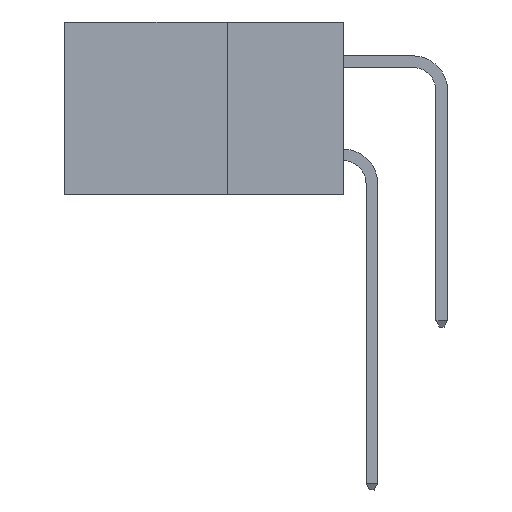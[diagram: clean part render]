
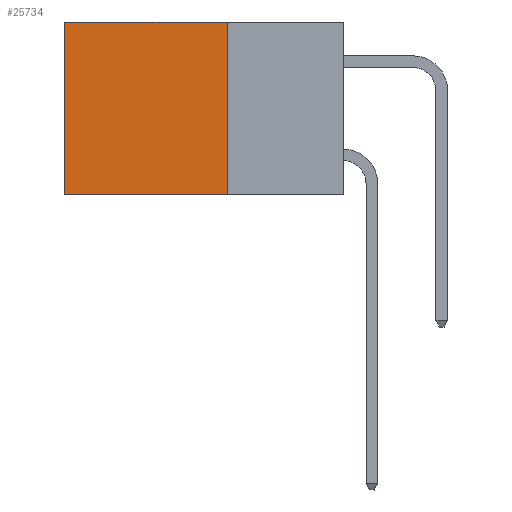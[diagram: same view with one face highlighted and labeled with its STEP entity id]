
A CAD part, left-side view. The second image highlights one B-rep face of the part: STEP entity #25734.
In plain terms, the highlighted planar face has unit normal (-1, 0, 0).
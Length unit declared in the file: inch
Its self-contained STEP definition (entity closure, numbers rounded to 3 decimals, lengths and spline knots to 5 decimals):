
#256 = CARTESIAN_POINT ( 'NONE',  ( 0.298, 0.25, -0.37 ) ) ;
#2157 = CARTESIAN_POINT ( 'NONE',  ( 0.298, 0.6, 0. ) ) ;
#3060 = LINE ( 'NONE', #29448, #22482 ) ;
#4699 = AXIS2_PLACEMENT_3D ( 'NONE', #28687, #28390, #28597 ) ;
#5177 = CARTESIAN_POINT ( 'NONE',  ( 0.298, 0.6, 0. ) ) ;
#5462 = VECTOR ( 'NONE', #14297, 39.37008 ) ;
#5590 = VERTEX_POINT ( 'NONE', #5177 ) ;
#5733 = CARTESIAN_POINT ( 'NONE',  ( 0.298, 0.25, 0. ) ) ;
#6055 = EDGE_CURVE ( 'NONE', #10952, #9444, #3060, .T. ) ;
#7661 = VERTEX_POINT ( 'NONE', #23464 ) ;
#8648 = LINE ( 'NONE', #2157, #25894 ) ;
#9320 = EDGE_LOOP ( 'NONE', ( #13566, #17586, #14301, #10245 ) ) ;
#9444 = VERTEX_POINT ( 'NONE', #256 ) ;
#10245 = ORIENTED_EDGE ( 'NONE', *, *, #13173, .T. ) ;
#10952 = VERTEX_POINT ( 'NONE', #5733 ) ;
#12190 = CARTESIAN_POINT ( 'NONE',  ( 0.298, 0.25, 0. ) ) ;
#12520 = PLANE ( 'NONE',  #4699 ) ;
#13173 = EDGE_CURVE ( 'NONE', #10952, #5590, #18388, .T. ) ;
#13566 = ORIENTED_EDGE ( 'NONE', *, *, #13704, .T. ) ;
#13704 = EDGE_CURVE ( 'NONE', #5590, #7661, #8648, .T. ) ;
#14297 = DIRECTION ( 'NONE',  ( 0., 1., 0. ) ) ;
#14301 = ORIENTED_EDGE ( 'NONE', *, *, #6055, .F. ) ;
#14384 = EDGE_CURVE ( 'NONE', #9444, #7661, #21208, .T. ) ;
#15208 = FACE_OUTER_BOUND ( 'NONE', #9320, .T. ) ;
#16207 = CARTESIAN_POINT ( 'NONE',  ( 0.298, 0.25, -0.37 ) ) ;
#17586 = ORIENTED_EDGE ( 'NONE', *, *, #14384, .F. ) ;
#18014 = DIRECTION ( 'NONE',  ( 0., 0., -1. ) ) ;
#18388 = LINE ( 'NONE', #12190, #5462 ) ;
#21208 = LINE ( 'NONE', #16207, #26947 ) ;
#22482 = VECTOR ( 'NONE', #18014, 39.37008 ) ;
#23464 = CARTESIAN_POINT ( 'NONE',  ( 0.298, 0.6, -0.37 ) ) ;
#25734 = ADVANCED_FACE ( 'NONE', ( #15208 ), #12520, .F. ) ;
#25894 = VECTOR ( 'NONE', #26279, 39.37008 ) ;
#26279 = DIRECTION ( 'NONE',  ( 0., 0., -1. ) ) ;
#26947 = VECTOR ( 'NONE', #29625, 39.37008 ) ;
#28390 = DIRECTION ( 'NONE',  ( 1., 0., 0. ) ) ;
#28597 = DIRECTION ( 'NONE',  ( 0., 0., -1. ) ) ;
#28687 = CARTESIAN_POINT ( 'NONE',  ( 0.298, 0.25, 0. ) ) ;
#29448 = CARTESIAN_POINT ( 'NONE',  ( 0.298, 0.25, 0. ) ) ;
#29625 = DIRECTION ( 'NONE',  ( 0., 1., 0. ) ) ;
